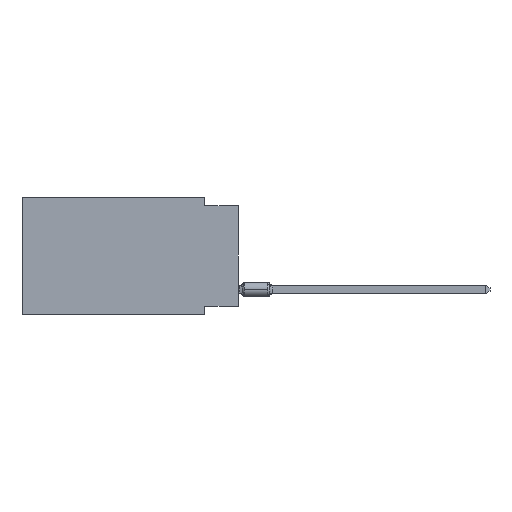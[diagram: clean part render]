
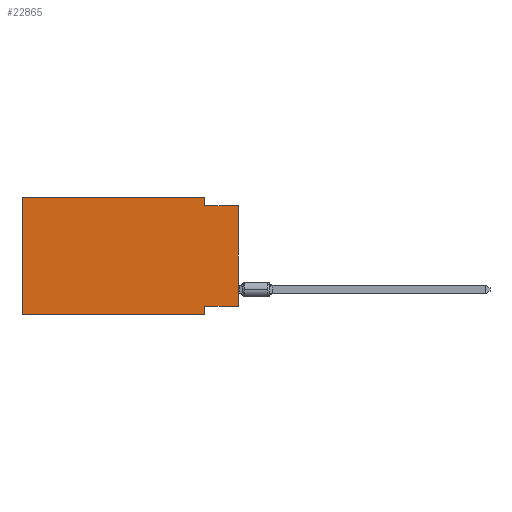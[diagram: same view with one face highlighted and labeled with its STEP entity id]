
A CAD part, left-side view. The second image highlights one B-rep face of the part: STEP entity #22865.
In plain terms, the highlighted planar face has unit normal (-1, 0, 0).
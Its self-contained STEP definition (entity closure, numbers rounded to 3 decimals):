
#517 = CARTESIAN_POINT ( 'NONE',  ( 0., 16.383, 0. ) ) ;
#815 = LINE ( 'NONE', #26424, #4347 ) ;
#1091 = DIRECTION ( 'NONE',  ( 0., 1., 0. ) ) ;
#1142 = FACE_OUTER_BOUND ( 'NONE', #27057, .T. ) ;
#1506 = CARTESIAN_POINT ( 'NONE',  ( 0., 2.54, -8.89 ) ) ;
#1946 = EDGE_CURVE ( 'NONE', #26946, #7258, #27246, .T. ) ;
#2582 = ORIENTED_EDGE ( 'NONE', *, *, #8693, .F. ) ;
#2856 = CARTESIAN_POINT ( 'NONE',  ( 0., 0., -0.635 ) ) ;
#3084 = PLANE ( 'NONE',  #26202 ) ;
#3360 = DIRECTION ( 'NONE',  ( 1., 0., 0. ) ) ;
#4295 = LINE ( 'NONE', #18714, #25285 ) ;
#4347 = VECTOR ( 'NONE', #1091, 1000. ) ;
#4388 = DIRECTION ( 'NONE',  ( 0., 0., -1. ) ) ;
#5635 = DIRECTION ( 'NONE',  ( 0., -1., 0. ) ) ;
#5685 = ORIENTED_EDGE ( 'NONE', *, *, #19218, .F. ) ;
#5841 = CARTESIAN_POINT ( 'NONE',  ( 0., 2.54, 0. ) ) ;
#6237 = ORIENTED_EDGE ( 'NONE', *, *, #13495, .F. ) ;
#6270 = VERTEX_POINT ( 'NONE', #18849 ) ;
#6737 = VECTOR ( 'NONE', #5635, 1000. ) ;
#7258 = VERTEX_POINT ( 'NONE', #1506 ) ;
#7577 = VERTEX_POINT ( 'NONE', #11886 ) ;
#8642 = CARTESIAN_POINT ( 'NONE',  ( 0., 0., -0.635 ) ) ;
#8693 = EDGE_CURVE ( 'NONE', #18854, #7577, #22463, .T. ) ;
#9093 = EDGE_CURVE ( 'NONE', #6270, #10830, #10647, .T. ) ;
#9219 = VECTOR ( 'NONE', #16239, 1000. ) ;
#9713 = ORIENTED_EDGE ( 'NONE', *, *, #10422, .F. ) ;
#10201 = CARTESIAN_POINT ( 'NONE',  ( 0., 16.383, -8.89 ) ) ;
#10422 = EDGE_CURVE ( 'NONE', #15195, #26946, #815, .T. ) ;
#10647 = LINE ( 'NONE', #517, #16241 ) ;
#10830 = VERTEX_POINT ( 'NONE', #15278 ) ;
#10881 = VERTEX_POINT ( 'NONE', #8642 ) ;
#10917 = CARTESIAN_POINT ( 'NONE',  ( 0., 2.54, -8.89 ) ) ;
#11129 = CARTESIAN_POINT ( 'NONE',  ( 0., 0., -8.255 ) ) ;
#11305 = DIRECTION ( 'NONE',  ( 0., -1., 0. ) ) ;
#11527 = DIRECTION ( 'NONE',  ( 0., 0., -1. ) ) ;
#11886 = CARTESIAN_POINT ( 'NONE',  ( 0., 2.54, -0.635 ) ) ;
#12236 = CARTESIAN_POINT ( 'NONE',  ( 0., 0., 0. ) ) ;
#13068 = ORIENTED_EDGE ( 'NONE', *, *, #17692, .T. ) ;
#13495 = EDGE_CURVE ( 'NONE', #7577, #10881, #15186, .T. ) ;
#13877 = ORIENTED_EDGE ( 'NONE', *, *, #1946, .F. ) ;
#14311 = LINE ( 'NONE', #12236, #21385 ) ;
#15186 = LINE ( 'NONE', #2856, #23975 ) ;
#15195 = VERTEX_POINT ( 'NONE', #11129 ) ;
#15278 = CARTESIAN_POINT ( 'NONE',  ( 0., 16.383, 0. ) ) ;
#15536 = ORIENTED_EDGE ( 'NONE', *, *, #16204, .T. ) ;
#16087 = CARTESIAN_POINT ( 'NONE',  ( 0., 2.54, -8.255 ) ) ;
#16204 = EDGE_CURVE ( 'NONE', #6270, #7258, #18516, .T. ) ;
#16239 = DIRECTION ( 'NONE',  ( 0., 0., -1. ) ) ;
#16241 = VECTOR ( 'NONE', #19247, 1000. ) ;
#17692 = EDGE_CURVE ( 'NONE', #15195, #10881, #14311, .T. ) ;
#18516 = LINE ( 'NONE', #10201, #6737 ) ;
#18714 = CARTESIAN_POINT ( 'NONE',  ( 0., 16.383, 0. ) ) ;
#18849 = CARTESIAN_POINT ( 'NONE',  ( 0., 16.383, -8.89 ) ) ;
#18854 = VERTEX_POINT ( 'NONE', #27031 ) ;
#19218 = EDGE_CURVE ( 'NONE', #10830, #18854, #4295, .T. ) ;
#19247 = DIRECTION ( 'NONE',  ( 0., 0., 1. ) ) ;
#19974 = CARTESIAN_POINT ( 'NONE',  ( 0., 16.383, 0. ) ) ;
#21059 = VECTOR ( 'NONE', #4388, 1000. ) ;
#21385 = VECTOR ( 'NONE', #22739, 1000. ) ;
#22463 = LINE ( 'NONE', #5841, #9219 ) ;
#22739 = DIRECTION ( 'NONE',  ( 0., 0., 1. ) ) ;
#22865 = ADVANCED_FACE ( 'NONE', ( #1142 ), #3084, .F. ) ;
#23975 = VECTOR ( 'NONE', #11305, 1000. ) ;
#24559 = ORIENTED_EDGE ( 'NONE', *, *, #9093, .F. ) ;
#25285 = VECTOR ( 'NONE', #25354, 1000. ) ;
#25354 = DIRECTION ( 'NONE',  ( 0., -1., 0. ) ) ;
#26202 = AXIS2_PLACEMENT_3D ( 'NONE', #19974, #3360, #11527 ) ;
#26424 = CARTESIAN_POINT ( 'NONE',  ( 0., 0., -8.255 ) ) ;
#26946 = VERTEX_POINT ( 'NONE', #16087 ) ;
#27031 = CARTESIAN_POINT ( 'NONE',  ( 0., 2.54, 0. ) ) ;
#27057 = EDGE_LOOP ( 'NONE', ( #13068, #6237, #2582, #5685, #24559, #15536, #13877, #9713 ) ) ;
#27246 = LINE ( 'NONE', #10917, #21059 ) ;
